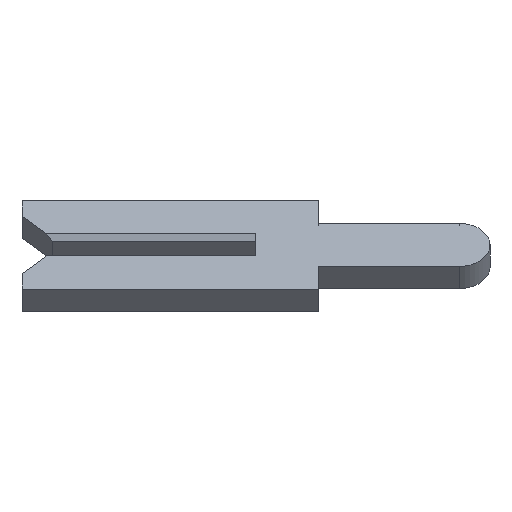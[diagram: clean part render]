
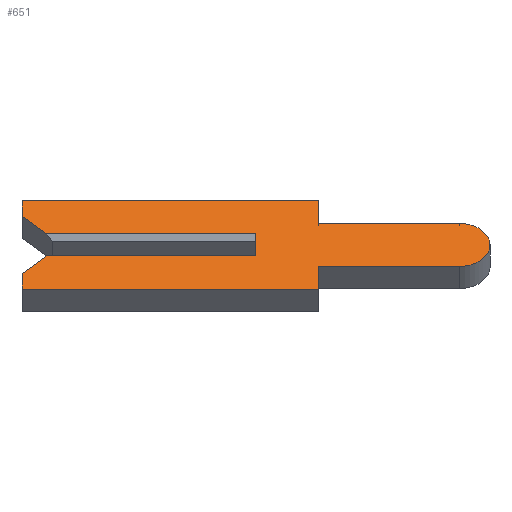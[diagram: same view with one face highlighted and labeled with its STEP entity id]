
A CAD part, left-side view. The second image highlights one B-rep face of the part: STEP entity #651.
In plain terms, the highlighted face is planar.
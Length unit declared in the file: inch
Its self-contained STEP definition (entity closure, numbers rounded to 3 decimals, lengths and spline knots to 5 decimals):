
#14 = LINE ( 'NONE', #415, #807 ) ;
#19 = LINE ( 'NONE', #363, #973 ) ;
#21 = EDGE_CURVE ( 'NONE', #77, #99, #339, .T. ) ;
#27 = EDGE_CURVE ( 'NONE', #223, #77, #438, .T. ) ;
#31 = CARTESIAN_POINT ( 'NONE',  ( -0.01, 0.15, -0.026 ) ) ;
#40 = LINE ( 'NONE', #1007, #914 ) ;
#74 = LINE ( 'NONE', #964, #840 ) ;
#77 = VERTEX_POINT ( 'NONE', #334 ) ;
#79 = AXIS2_PLACEMENT_3D ( 'NONE', #586, #808, #254 ) ;
#85 = VECTOR ( 'NONE', #910, 39.37008 ) ;
#87 = CIRCLE ( 'NONE', #79, 0.0195 ) ;
#89 = DIRECTION ( 'NONE',  ( 0., -1., 0. ) ) ;
#90 = DIRECTION ( 'NONE',  ( 0., 0., -1. ) ) ;
#95 = CARTESIAN_POINT ( 'NONE',  ( -0.01, -0.04, -0.0195 ) ) ;
#99 = VERTEX_POINT ( 'NONE', #498 ) ;
#103 = DIRECTION ( 'NONE',  ( 0., 0., 1. ) ) ;
#104 = EDGE_CURVE ( 'NONE', #202, #588, #14, .T. ) ;
#113 = CARTESIAN_POINT ( 'NONE',  ( -0.01, 0., -0.01 ) ) ;
#126 = VECTOR ( 'NONE', #736, 39.37008 ) ;
#163 = CARTESIAN_POINT ( 'NONE',  ( -0.01, -0.1305, -0.0195 ) ) ;
#167 = DIRECTION ( 'NONE',  ( 0., 1., 0. ) ) ;
#170 = VERTEX_POINT ( 'NONE', #979 ) ;
#173 = EDGE_CURVE ( 'NONE', #468, #202, #87, .T. ) ;
#175 = LINE ( 'NONE', #406, #484 ) ;
#179 = VERTEX_POINT ( 'NONE', #31 ) ;
#181 = ORIENTED_EDGE ( 'NONE', *, *, #104, .F. ) ;
#202 = VERTEX_POINT ( 'NONE', #163 ) ;
#221 = CARTESIAN_POINT ( 'NONE',  ( -0.01, 0., 0.01 ) ) ;
#223 = VERTEX_POINT ( 'NONE', #745 ) ;
#227 = LINE ( 'NONE', #327, #557 ) ;
#232 = VECTOR ( 'NONE', #89, 39.37008 ) ;
#243 = LINE ( 'NONE', #666, #831 ) ;
#254 = DIRECTION ( 'NONE',  ( 0., 0., -1. ) ) ;
#256 = DIRECTION ( 'NONE',  ( 0., 1., 0. ) ) ;
#257 = LINE ( 'NONE', #988, #560 ) ;
#258 = CARTESIAN_POINT ( 'NONE',  ( -0.01, -0.04, -0.04 ) ) ;
#275 = ORIENTED_EDGE ( 'NONE', *, *, #27, .F. ) ;
#277 = EDGE_CURVE ( 'NONE', #631, #707, #243, .T. ) ;
#289 = VECTOR ( 'NONE', #881, 39.37008 ) ;
#301 = PLANE ( 'NONE',  #581 ) ;
#304 = VERTEX_POINT ( 'NONE', #258 ) ;
#314 = VECTOR ( 'NONE', #103, 39.37008 ) ;
#327 = CARTESIAN_POINT ( 'NONE',  ( -0.01, 0.1305, 0.0065 ) ) ;
#334 = CARTESIAN_POINT ( 'NONE',  ( -0.01, -0.04, 0.04 ) ) ;
#335 = EDGE_CURVE ( 'NONE', #170, #345, #587, .T. ) ;
#339 = LINE ( 'NONE', #888, #289 ) ;
#344 = CARTESIAN_POINT ( 'NONE',  ( -0.01, -0.1305, -0.01 ) ) ;
#345 = VERTEX_POINT ( 'NONE', #113 ) ;
#353 = EDGE_CURVE ( 'NONE', #99, #468, #257, .T. ) ;
#357 = LINE ( 'NONE', #589, #314 ) ;
#363 = CARTESIAN_POINT ( 'NONE',  ( -0.01, 0., 0.0065 ) ) ;
#375 = DIRECTION ( 'NONE',  ( 0., 0., -1. ) ) ;
#378 = CARTESIAN_POINT ( 'NONE',  ( -0.01, -0.1305, 0.0195 ) ) ;
#388 = EDGE_CURVE ( 'NONE', #418, #179, #357, .T. ) ;
#393 = EDGE_LOOP ( 'NONE', ( #709, #999, #835, #922, #403, #981, #533, #181, #829, #958, #441, #275, #432, #526 ) ) ;
#403 = ORIENTED_EDGE ( 'NONE', *, *, #388, .F. ) ;
#406 = CARTESIAN_POINT ( 'NONE',  ( -0.01, 0.15, -0.04 ) ) ;
#415 = CARTESIAN_POINT ( 'NONE',  ( -0.01, -0.04, -0.0195 ) ) ;
#418 = VERTEX_POINT ( 'NONE', #652 ) ;
#428 = DIRECTION ( 'NONE',  ( 0., -1., 0. ) ) ;
#432 = ORIENTED_EDGE ( 'NONE', *, *, #838, .F. ) ;
#438 = LINE ( 'NONE', #963, #232 ) ;
#441 = ORIENTED_EDGE ( 'NONE', *, *, #21, .F. ) ;
#468 = VERTEX_POINT ( 'NONE', #378 ) ;
#484 = VECTOR ( 'NONE', #256, 39.37008 ) ;
#498 = CARTESIAN_POINT ( 'NONE',  ( -0.01, -0.04, 0.0195 ) ) ;
#499 = CARTESIAN_POINT ( 'NONE',  ( -0.01, 0.134, 0.01 ) ) ;
#507 = EDGE_CURVE ( 'NONE', #179, #170, #585, .T. ) ;
#526 = ORIENTED_EDGE ( 'NONE', *, *, #900, .F. ) ;
#533 = ORIENTED_EDGE ( 'NONE', *, *, #538, .F. ) ;
#538 = EDGE_CURVE ( 'NONE', #588, #304, #74, .T. ) ;
#557 = VECTOR ( 'NONE', #738, 39.37008 ) ;
#560 = VECTOR ( 'NONE', #428, 39.37008 ) ;
#581 = AXIS2_PLACEMENT_3D ( 'NONE', #855, #1012, #375 ) ;
#585 = LINE ( 'NONE', #959, #126 ) ;
#586 = CARTESIAN_POINT ( 'NONE',  ( -0.01, -0.1305, 0. ) ) ;
#587 = LINE ( 'NONE', #344, #85 ) ;
#588 = VERTEX_POINT ( 'NONE', #95 ) ;
#589 = CARTESIAN_POINT ( 'NONE',  ( -0.01, 0.15, -0.026 ) ) ;
#615 = EDGE_CURVE ( 'NONE', #304, #418, #175, .T. ) ;
#622 = VERTEX_POINT ( 'NONE', #667 ) ;
#631 = VERTEX_POINT ( 'NONE', #499 ) ;
#651 = ADVANCED_FACE ( 'NONE', ( #1021 ), #301, .F. ) ;
#652 = CARTESIAN_POINT ( 'NONE',  ( -0.01, 0.15, -0.04 ) ) ;
#666 = CARTESIAN_POINT ( 'NONE',  ( -0.01, 0.15, 0.01 ) ) ;
#667 = CARTESIAN_POINT ( 'NONE',  ( -0.01, 0.15, 0.026 ) ) ;
#703 = DIRECTION ( 'NONE',  ( 0., 0., 1. ) ) ;
#707 = VERTEX_POINT ( 'NONE', #221 ) ;
#709 = ORIENTED_EDGE ( 'NONE', *, *, #277, .T. ) ;
#736 = DIRECTION ( 'NONE',  ( 0., -0.707, 0.707 ) ) ;
#738 = DIRECTION ( 'NONE',  ( 0., 0.707, 0.707 ) ) ;
#743 = EDGE_CURVE ( 'NONE', #345, #707, #19, .T. ) ;
#745 = CARTESIAN_POINT ( 'NONE',  ( -0.01, 0.15, 0.04 ) ) ;
#807 = VECTOR ( 'NONE', #167, 39.37008 ) ;
#808 = DIRECTION ( 'NONE',  ( 1., 0., 0. ) ) ;
#829 = ORIENTED_EDGE ( 'NONE', *, *, #173, .F. ) ;
#831 = VECTOR ( 'NONE', #972, 39.37008 ) ;
#835 = ORIENTED_EDGE ( 'NONE', *, *, #335, .F. ) ;
#838 = EDGE_CURVE ( 'NONE', #622, #223, #40, .T. ) ;
#840 = VECTOR ( 'NONE', #90, 39.37008 ) ;
#855 = CARTESIAN_POINT ( 'NONE',  ( -0.01, -0.1305, 0. ) ) ;
#881 = DIRECTION ( 'NONE',  ( 0., 0., -1. ) ) ;
#888 = CARTESIAN_POINT ( 'NONE',  ( -0.01, -0.04, 0.04 ) ) ;
#900 = EDGE_CURVE ( 'NONE', #631, #622, #227, .T. ) ;
#910 = DIRECTION ( 'NONE',  ( 0., -1., 0. ) ) ;
#914 = VECTOR ( 'NONE', #703, 39.37008 ) ;
#922 = ORIENTED_EDGE ( 'NONE', *, *, #507, .F. ) ;
#939 = DIRECTION ( 'NONE',  ( 0., 0., 1. ) ) ;
#958 = ORIENTED_EDGE ( 'NONE', *, *, #353, .F. ) ;
#959 = CARTESIAN_POINT ( 'NONE',  ( -0.01, 0.1305, -0.0065 ) ) ;
#963 = CARTESIAN_POINT ( 'NONE',  ( -0.01, 0.15, 0.04 ) ) ;
#964 = CARTESIAN_POINT ( 'NONE',  ( -0.01, -0.04, -0.04 ) ) ;
#972 = DIRECTION ( 'NONE',  ( 0., -1., 0. ) ) ;
#973 = VECTOR ( 'NONE', #939, 39.37008 ) ;
#979 = CARTESIAN_POINT ( 'NONE',  ( -0.01, 0.134, -0.01 ) ) ;
#981 = ORIENTED_EDGE ( 'NONE', *, *, #615, .F. ) ;
#988 = CARTESIAN_POINT ( 'NONE',  ( -0.01, -0.04, 0.0195 ) ) ;
#999 = ORIENTED_EDGE ( 'NONE', *, *, #743, .F. ) ;
#1007 = CARTESIAN_POINT ( 'NONE',  ( -0.01, 0.15, 0.026 ) ) ;
#1012 = DIRECTION ( 'NONE',  ( 1., 0., 0. ) ) ;
#1021 = FACE_OUTER_BOUND ( 'NONE', #393, .T. ) ;
